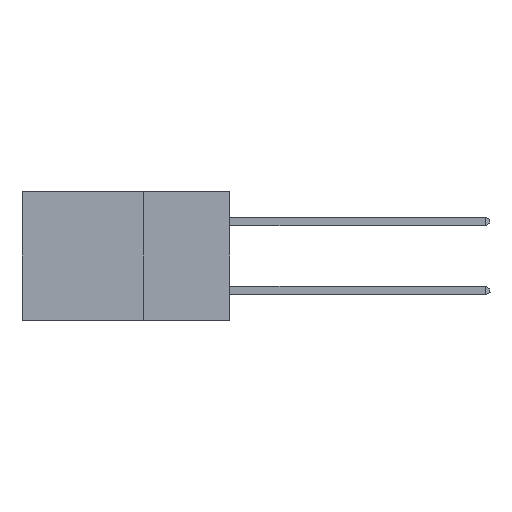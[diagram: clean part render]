
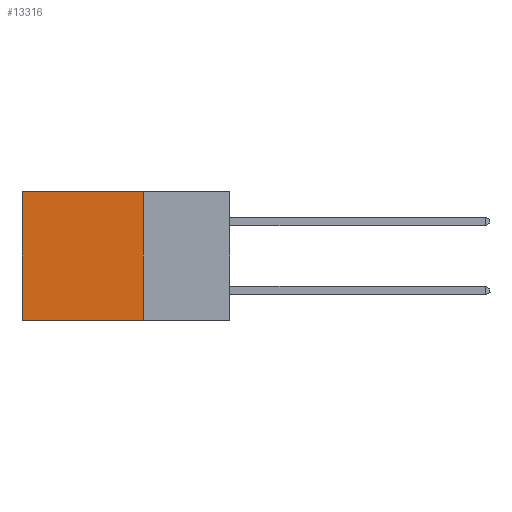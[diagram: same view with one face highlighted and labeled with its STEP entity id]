
A CAD part, left-side view. The second image highlights one B-rep face of the part: STEP entity #13316.
In plain terms, the highlighted planar face has unit normal (-1, 0, 0).
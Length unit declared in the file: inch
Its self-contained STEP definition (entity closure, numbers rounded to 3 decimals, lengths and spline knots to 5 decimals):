
#115 = DIRECTION ( 'NONE',  ( 1., 0., 0. ) ) ;
#599 = DIRECTION ( 'NONE',  ( 0., 0., -1. ) ) ;
#1031 = VERTEX_POINT ( 'NONE', #19526 ) ;
#1710 = LINE ( 'NONE', #15229, #19197 ) ;
#3358 = EDGE_CURVE ( 'NONE', #11362, #1031, #12840, .T. ) ;
#3380 = EDGE_CURVE ( 'NONE', #1031, #6524, #1710, .T. ) ;
#3641 = DIRECTION ( 'NONE',  ( 0., 0., -1. ) ) ;
#4810 = VECTOR ( 'NONE', #8699, 39.37008 ) ;
#4833 = EDGE_CURVE ( 'NONE', #11362, #8216, #19410, .T. ) ;
#5781 = EDGE_LOOP ( 'NONE', ( #13869, #14848, #7941, #8301 ) ) ;
#6524 = VERTEX_POINT ( 'NONE', #15269 ) ;
#6888 = CARTESIAN_POINT ( 'NONE',  ( 0.298, 0.25, 0. ) ) ;
#7676 = CARTESIAN_POINT ( 'NONE',  ( 0.298, 0.6, 0. ) ) ;
#7941 = ORIENTED_EDGE ( 'NONE', *, *, #3358, .F. ) ;
#8216 = VERTEX_POINT ( 'NONE', #12407 ) ;
#8301 = ORIENTED_EDGE ( 'NONE', *, *, #4833, .T. ) ;
#8303 = DIRECTION ( 'NONE',  ( 0., 0., -1. ) ) ;
#8609 = LINE ( 'NONE', #7676, #20054 ) ;
#8699 = DIRECTION ( 'NONE',  ( 0., 1., 0. ) ) ;
#9111 = CARTESIAN_POINT ( 'NONE',  ( 0.298, 0.25, 0. ) ) ;
#10044 = CARTESIAN_POINT ( 'NONE',  ( 0.298, 0.25, 0. ) ) ;
#11362 = VERTEX_POINT ( 'NONE', #9111 ) ;
#11809 = CARTESIAN_POINT ( 'NONE',  ( 0.298, 0.25, 0. ) ) ;
#11993 = EDGE_CURVE ( 'NONE', #8216, #6524, #8609, .T. ) ;
#12407 = CARTESIAN_POINT ( 'NONE',  ( 0.298, 0.6, 0. ) ) ;
#12840 = LINE ( 'NONE', #11809, #21386 ) ;
#13059 = FACE_OUTER_BOUND ( 'NONE', #5781, .T. ) ;
#13316 = ADVANCED_FACE ( 'NONE', ( #13059 ), #18530, .F. ) ;
#13869 = ORIENTED_EDGE ( 'NONE', *, *, #11993, .T. ) ;
#14848 = ORIENTED_EDGE ( 'NONE', *, *, #3380, .F. ) ;
#15229 = CARTESIAN_POINT ( 'NONE',  ( 0.298, 0.25, -0.37 ) ) ;
#15269 = CARTESIAN_POINT ( 'NONE',  ( 0.298, 0.6, -0.37 ) ) ;
#18530 = PLANE ( 'NONE',  #20585 ) ;
#18630 = DIRECTION ( 'NONE',  ( 0., 1., 0. ) ) ;
#19197 = VECTOR ( 'NONE', #18630, 39.37008 ) ;
#19410 = LINE ( 'NONE', #6888, #4810 ) ;
#19526 = CARTESIAN_POINT ( 'NONE',  ( 0.298, 0.25, -0.37 ) ) ;
#20054 = VECTOR ( 'NONE', #599, 39.37008 ) ;
#20585 = AXIS2_PLACEMENT_3D ( 'NONE', #10044, #115, #8303 ) ;
#21386 = VECTOR ( 'NONE', #3641, 39.37008 ) ;
